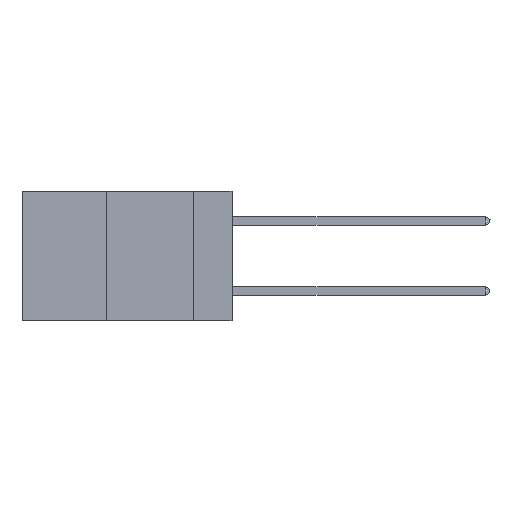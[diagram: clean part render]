
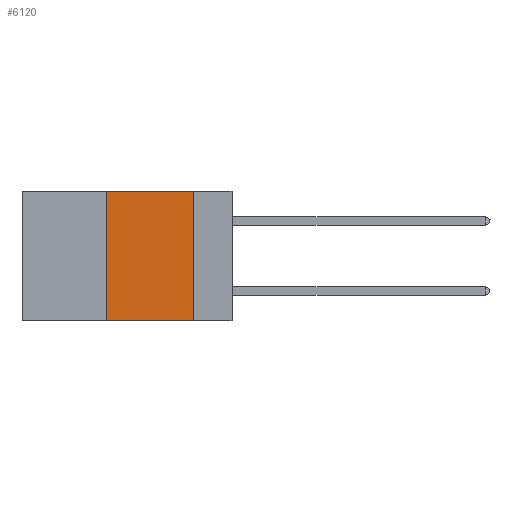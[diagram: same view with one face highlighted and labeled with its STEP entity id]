
A CAD part, left-side view. The second image highlights one B-rep face of the part: STEP entity #6120.
In plain terms, the highlighted planar face has unit normal (-1, 0, 0).
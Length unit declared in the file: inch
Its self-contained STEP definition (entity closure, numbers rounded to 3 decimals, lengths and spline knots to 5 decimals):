
#8 = CARTESIAN_POINT ( 'NONE',  ( 0., 0.11, 0. ) ) ;
#571 = CARTESIAN_POINT ( 'NONE',  ( 0., 0.6, 0. ) ) ;
#704 = ORIENTED_EDGE ( 'NONE', *, *, #5392, .F. ) ;
#840 = DIRECTION ( 'NONE',  ( 0., -1., 0. ) ) ;
#1745 = CARTESIAN_POINT ( 'NONE',  ( 0., 0.11, -0.37 ) ) ;
#1984 = DIRECTION ( 'NONE',  ( 0., 0., 1. ) ) ;
#2337 = EDGE_CURVE ( 'NONE', #2883, #8544, #16220, .T. ) ;
#2871 = AXIS2_PLACEMENT_3D ( 'NONE', #8338, #18703, #9868 ) ;
#2883 = VERTEX_POINT ( 'NONE', #3665 ) ;
#3337 = VECTOR ( 'NONE', #12699, 39.37008 ) ;
#3632 = LINE ( 'NONE', #9620, #18598 ) ;
#3665 = CARTESIAN_POINT ( 'NONE',  ( 0., 0.36, -0.37 ) ) ;
#5392 = EDGE_CURVE ( 'NONE', #2883, #18750, #3632, .T. ) ;
#6120 = ADVANCED_FACE ( 'NONE', ( #10030 ), #11318, .F. ) ;
#7051 = EDGE_CURVE ( 'NONE', #19150, #8544, #14001, .T. ) ;
#7818 = ORIENTED_EDGE ( 'NONE', *, *, #9981, .F. ) ;
#7851 = LINE ( 'NONE', #571, #3337 ) ;
#8338 = CARTESIAN_POINT ( 'NONE',  ( 0., 0.6, 0. ) ) ;
#8544 = VERTEX_POINT ( 'NONE', #1745 ) ;
#9620 = CARTESIAN_POINT ( 'NONE',  ( 0., 0.36, 0. ) ) ;
#9868 = DIRECTION ( 'NONE',  ( 0., 0., -1. ) ) ;
#9981 = EDGE_CURVE ( 'NONE', #18750, #19150, #7851, .T. ) ;
#10030 = FACE_OUTER_BOUND ( 'NONE', #13741, .T. ) ;
#11318 = PLANE ( 'NONE',  #2871 ) ;
#11456 = CARTESIAN_POINT ( 'NONE',  ( 0., 0.6, -0.37 ) ) ;
#12097 = CARTESIAN_POINT ( 'NONE',  ( 0., 0.11, 0. ) ) ;
#12699 = DIRECTION ( 'NONE',  ( 0., -1., 0. ) ) ;
#13434 = ORIENTED_EDGE ( 'NONE', *, *, #7051, .F. ) ;
#13741 = EDGE_LOOP ( 'NONE', ( #13434, #7818, #704, #15605 ) ) ;
#14001 = LINE ( 'NONE', #8, #17853 ) ;
#15605 = ORIENTED_EDGE ( 'NONE', *, *, #2337, .T. ) ;
#16220 = LINE ( 'NONE', #11456, #16658 ) ;
#16541 = DIRECTION ( 'NONE',  ( 0., 0., -1. ) ) ;
#16658 = VECTOR ( 'NONE', #840, 39.37008 ) ;
#17853 = VECTOR ( 'NONE', #16541, 39.37008 ) ;
#18135 = CARTESIAN_POINT ( 'NONE',  ( 0., 0.36, 0. ) ) ;
#18598 = VECTOR ( 'NONE', #1984, 39.37008 ) ;
#18703 = DIRECTION ( 'NONE',  ( 1., 0., 0. ) ) ;
#18750 = VERTEX_POINT ( 'NONE', #18135 ) ;
#19150 = VERTEX_POINT ( 'NONE', #12097 ) ;
